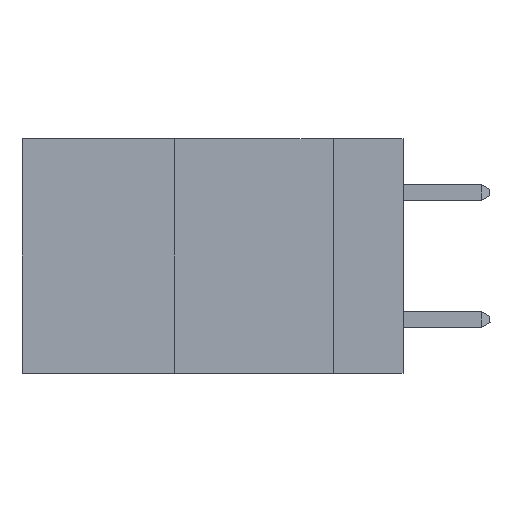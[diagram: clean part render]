
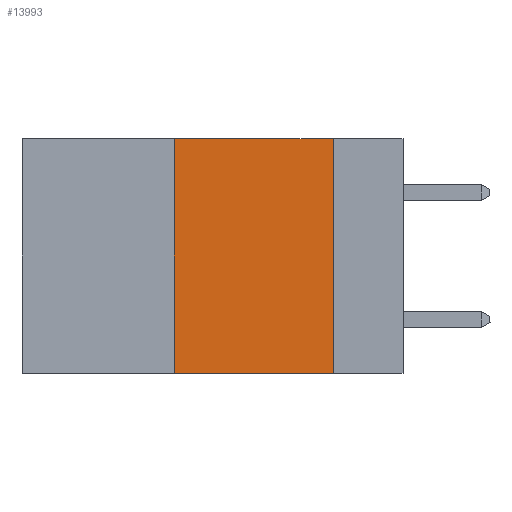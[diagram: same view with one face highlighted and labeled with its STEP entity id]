
A CAD part, left-side view. The second image highlights one B-rep face of the part: STEP entity #13993.
In plain terms, the highlighted planar face has unit normal (-1, 0, 0).
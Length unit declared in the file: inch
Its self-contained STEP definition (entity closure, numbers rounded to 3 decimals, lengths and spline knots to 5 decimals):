
#1295 = CARTESIAN_POINT ( 'NONE',  ( 0., 0.6, -0.37 ) ) ;
#1507 = DIRECTION ( 'NONE',  ( 0., 0., -1. ) ) ;
#1986 = ORIENTED_EDGE ( 'NONE', *, *, #3893, .F. ) ;
#2090 = VERTEX_POINT ( 'NONE', #7524 ) ;
#2402 = VERTEX_POINT ( 'NONE', #11455 ) ;
#2533 = DIRECTION ( 'NONE',  ( 0., -1., 0. ) ) ;
#3770 = CARTESIAN_POINT ( 'NONE',  ( 0., 0.36, 0. ) ) ;
#3893 = EDGE_CURVE ( 'NONE', #2090, #2402, #9104, .T. ) ;
#4002 = EDGE_CURVE ( 'NONE', #7568, #2402, #9768, .T. ) ;
#4776 = CARTESIAN_POINT ( 'NONE',  ( 0., 0.11, 0. ) ) ;
#5551 = VECTOR ( 'NONE', #2533, 39.37008 ) ;
#6574 = LINE ( 'NONE', #3770, #8548 ) ;
#6718 = ORIENTED_EDGE ( 'NONE', *, *, #4002, .T. ) ;
#7279 = DIRECTION ( 'NONE',  ( 1., 0., 0. ) ) ;
#7357 = ORIENTED_EDGE ( 'NONE', *, *, #9296, .F. ) ;
#7463 = EDGE_CURVE ( 'NONE', #7568, #15672, #6574, .T. ) ;
#7481 = CARTESIAN_POINT ( 'NONE',  ( 0., 0.6, 0. ) ) ;
#7524 = CARTESIAN_POINT ( 'NONE',  ( 0., 0.11, 0. ) ) ;
#7568 = VERTEX_POINT ( 'NONE', #18541 ) ;
#7771 = AXIS2_PLACEMENT_3D ( 'NONE', #7481, #7279, #11790 ) ;
#8081 = EDGE_LOOP ( 'NONE', ( #1986, #7357, #11863, #6718 ) ) ;
#8548 = VECTOR ( 'NONE', #9499, 39.37008 ) ;
#9104 = LINE ( 'NONE', #4776, #9874 ) ;
#9296 = EDGE_CURVE ( 'NONE', #15672, #2090, #13899, .T. ) ;
#9499 = DIRECTION ( 'NONE',  ( 0., 0., 1. ) ) ;
#9753 = CARTESIAN_POINT ( 'NONE',  ( 0., 0.36, 0. ) ) ;
#9768 = LINE ( 'NONE', #1295, #13483 ) ;
#9859 = DIRECTION ( 'NONE',  ( 0., -1., 0. ) ) ;
#9874 = VECTOR ( 'NONE', #1507, 39.37008 ) ;
#11455 = CARTESIAN_POINT ( 'NONE',  ( 0., 0.11, -0.37 ) ) ;
#11620 = FACE_OUTER_BOUND ( 'NONE', #8081, .T. ) ;
#11790 = DIRECTION ( 'NONE',  ( 0., 0., -1. ) ) ;
#11863 = ORIENTED_EDGE ( 'NONE', *, *, #7463, .F. ) ;
#13483 = VECTOR ( 'NONE', #9859, 39.37008 ) ;
#13810 = CARTESIAN_POINT ( 'NONE',  ( 0., 0.6, 0. ) ) ;
#13899 = LINE ( 'NONE', #13810, #5551 ) ;
#13993 = ADVANCED_FACE ( 'NONE', ( #11620 ), #15885, .F. ) ;
#15672 = VERTEX_POINT ( 'NONE', #9753 ) ;
#15885 = PLANE ( 'NONE',  #7771 ) ;
#18541 = CARTESIAN_POINT ( 'NONE',  ( 0., 0.36, -0.37 ) ) ;
